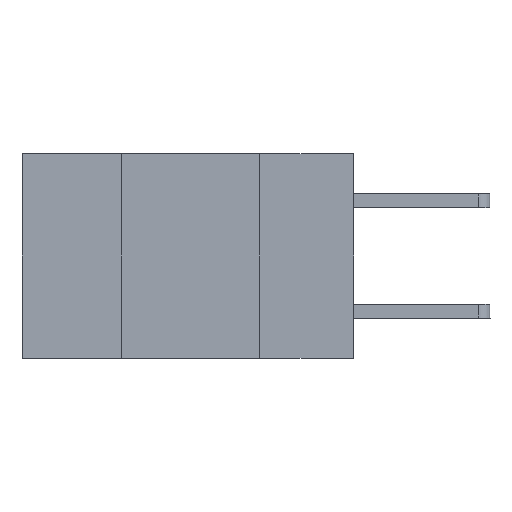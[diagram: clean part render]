
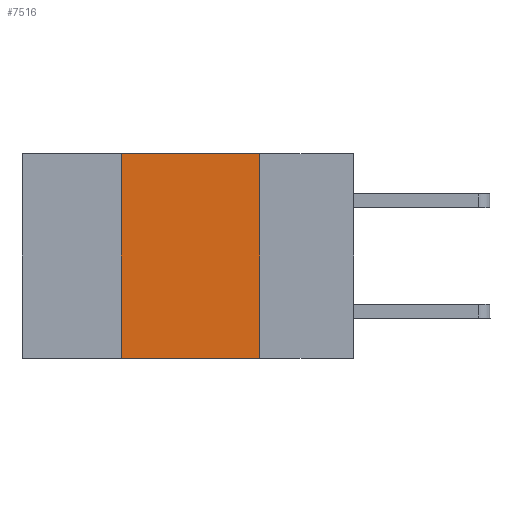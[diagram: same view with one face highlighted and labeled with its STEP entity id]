
A CAD part, left-side view. The second image highlights one B-rep face of the part: STEP entity #7516.
In plain terms, the highlighted planar face has unit normal (-1, 0, 0).
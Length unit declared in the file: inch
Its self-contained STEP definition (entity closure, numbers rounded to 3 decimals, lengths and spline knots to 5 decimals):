
#74 = PLANE ( 'NONE',  #6149 ) ;
#166 = CARTESIAN_POINT ( 'NONE',  ( 0., 0.17, 0. ) ) ;
#361 = EDGE_CURVE ( 'NONE', #7087, #5065, #4441, .T. ) ;
#839 = CARTESIAN_POINT ( 'NONE',  ( 0., 0.6, 0. ) ) ;
#886 = LINE ( 'NONE', #9346, #2191 ) ;
#952 = CARTESIAN_POINT ( 'NONE',  ( 0., 0.42, 0. ) ) ;
#1408 = DIRECTION ( 'NONE',  ( 0., -1., 0. ) ) ;
#1543 = DIRECTION ( 'NONE',  ( 0., 0., -1. ) ) ;
#1560 = EDGE_CURVE ( 'NONE', #2363, #5065, #886, .T. ) ;
#1796 = DIRECTION ( 'NONE',  ( 0., -1., 0. ) ) ;
#2191 = VECTOR ( 'NONE', #1408, 39.37008 ) ;
#2363 = VERTEX_POINT ( 'NONE', #7262 ) ;
#2890 = DIRECTION ( 'NONE',  ( 1., 0., 0. ) ) ;
#2896 = ORIENTED_EDGE ( 'NONE', *, *, #4277, .F. ) ;
#3077 = EDGE_LOOP ( 'NONE', ( #5665, #5311, #2896, #5453 ) ) ;
#3158 = VERTEX_POINT ( 'NONE', #3398 ) ;
#3398 = CARTESIAN_POINT ( 'NONE',  ( 0., 0.42, 0. ) ) ;
#3799 = LINE ( 'NONE', #7537, #8273 ) ;
#4277 = EDGE_CURVE ( 'NONE', #2363, #3158, #4554, .T. ) ;
#4441 = LINE ( 'NONE', #166, #7374 ) ;
#4454 = DIRECTION ( 'NONE',  ( 0., 0., 1. ) ) ;
#4554 = LINE ( 'NONE', #952, #7171 ) ;
#5065 = VERTEX_POINT ( 'NONE', #7927 ) ;
#5104 = FACE_OUTER_BOUND ( 'NONE', #3077, .T. ) ;
#5311 = ORIENTED_EDGE ( 'NONE', *, *, #5916, .F. ) ;
#5453 = ORIENTED_EDGE ( 'NONE', *, *, #1560, .T. ) ;
#5665 = ORIENTED_EDGE ( 'NONE', *, *, #361, .F. ) ;
#5916 = EDGE_CURVE ( 'NONE', #3158, #7087, #3799, .T. ) ;
#6149 = AXIS2_PLACEMENT_3D ( 'NONE', #839, #2890, #8768 ) ;
#7076 = CARTESIAN_POINT ( 'NONE',  ( 0., 0.17, 0. ) ) ;
#7087 = VERTEX_POINT ( 'NONE', #7076 ) ;
#7171 = VECTOR ( 'NONE', #4454, 39.37008 ) ;
#7262 = CARTESIAN_POINT ( 'NONE',  ( 0., 0.42, -0.37 ) ) ;
#7374 = VECTOR ( 'NONE', #1543, 39.37008 ) ;
#7516 = ADVANCED_FACE ( 'NONE', ( #5104 ), #74, .F. ) ;
#7537 = CARTESIAN_POINT ( 'NONE',  ( 0., 0.6, 0. ) ) ;
#7927 = CARTESIAN_POINT ( 'NONE',  ( 0., 0.17, -0.37 ) ) ;
#8273 = VECTOR ( 'NONE', #1796, 39.37008 ) ;
#8768 = DIRECTION ( 'NONE',  ( 0., 0., -1. ) ) ;
#9346 = CARTESIAN_POINT ( 'NONE',  ( 0., 0.6, -0.37 ) ) ;
